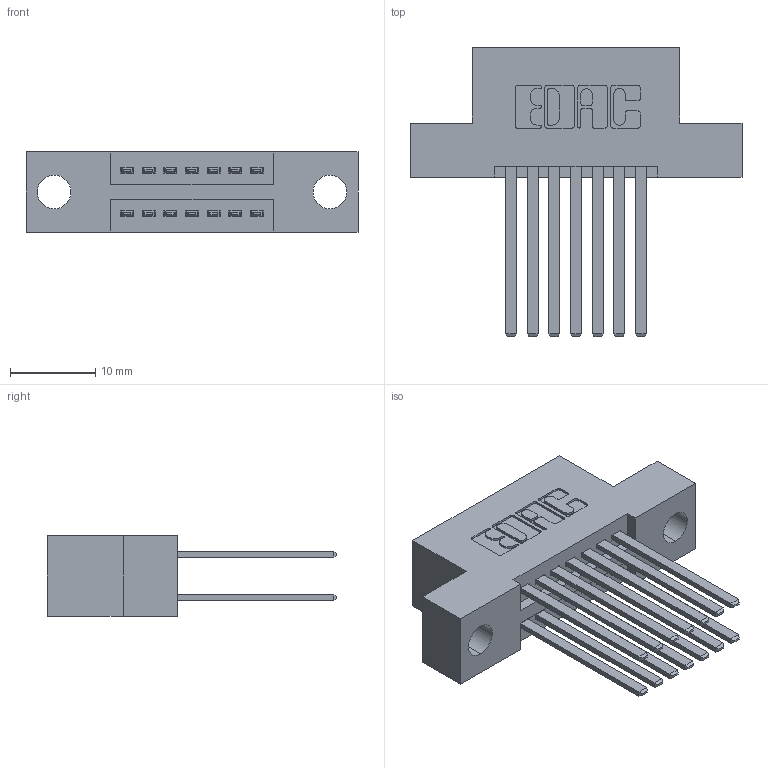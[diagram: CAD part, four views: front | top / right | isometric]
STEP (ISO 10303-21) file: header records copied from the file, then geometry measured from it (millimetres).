
FILE_DESCRIPTION (( 'STEP AP203' ), '1' );
FILE_NAME ('395-014-544-204.STEP', '2021-06-14T18:00:14', ( '' ), ( '' ), 'SwSTEP 2.0', 'SolidWorks 2020', '' );
FILE_SCHEMA (( 'CONFIG_CONTROL_DESIGN' ));
Length unit declared in the file: inch
Products named in the file (3): 345-292-001_345-293-144; 395-014-544-204; 345 Part_Flush Mounting Lugs - 0.156 Dia-TI
Assembly tree (15 placements, depth 2):
  395-014-544-204
    345 Part_Flush Mounting Lugs - 0.156 Dia-TI
    345-292-001_345-293-144  x14
Bounding box: 38.99 x 33.96 x 9.4 mm (x, y, z)
Volume: 3552.9 mm3; surface area: 5000.6 mm2
Topology: 15 solids, 15 shells, 756 faces, 2211 edges, 1454 vertices
Faces by surface type: plane 500, cylinder 256
Entity records: 10439 total; most frequent: CARTESIAN_POINT 1786, ORIENTED_EDGE 1718, DIRECTION 1615, EDGE_CURVE 859, VECTOR 703, LINE 703, VERTEX_POINT 570, AXIS2_PLACEMENT_3D 456
